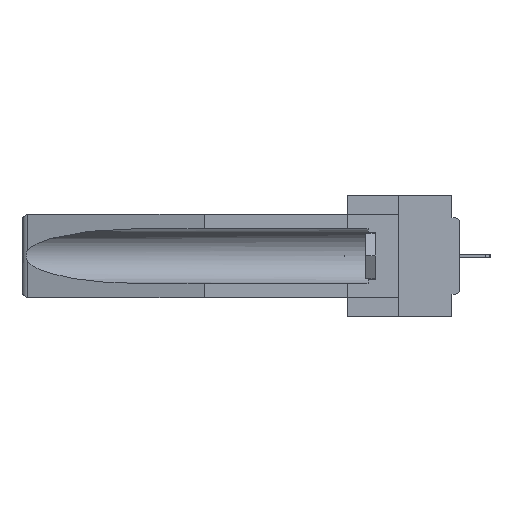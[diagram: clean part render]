
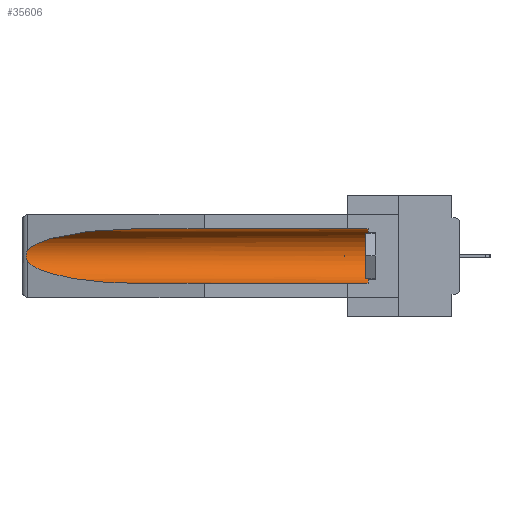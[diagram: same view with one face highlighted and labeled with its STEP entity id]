
A CAD part, left-side view. The second image highlights one B-rep face of the part: STEP entity #35606.
In plain terms, the highlighted cylindrical face has radius 2.857 mm (diameter 5.715 mm), a partial arc.
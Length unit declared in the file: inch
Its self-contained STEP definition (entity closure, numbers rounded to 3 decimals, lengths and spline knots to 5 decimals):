
#362 = ORIENTED_EDGE ( 'NONE', *, *, #18338, .F. ) ;
#703 = DIRECTION ( 'NONE',  ( 0., -1., 0. ) ) ;
#750 = CARTESIAN_POINT ( 'NONE',  ( 0.26537, 1.52718, -0.19328 ) ) ;
#1142 = DIRECTION ( 'NONE',  ( 0., 1., 0. ) ) ;
#1208 = DIRECTION ( 'NONE',  ( 0., 1., 0. ) ) ;
#2136 = EDGE_CURVE ( 'NONE', #2576, #16146, #40987, .T. ) ;
#2576 = VERTEX_POINT ( 'NONE', #750 ) ;
#3583 = CARTESIAN_POINT ( 'NONE',  ( 0.155, 0.126, -0.059 ) ) ;
#3843 = CARTESIAN_POINT ( 'NONE',  ( 0.25451, 1.48313, -0.24835 ) ) ;
#4377 = LINE ( 'NONE', #17209, #23886 ) ;
#4452 = CARTESIAN_POINT ( 'NONE',  ( 0.155, 1.07973, -0.284 ) ) ;
#5800 = CARTESIAN_POINT ( 'NONE',  ( 0.155, 1.07973, -0.059 ) ) ;
#6397 = ORIENTED_EDGE ( 'NONE', *, *, #2136, .T. ) ;
#6846 = EDGE_CURVE ( 'NONE', #24248, #17287, #15406, .T. ) ;
#8630 = CARTESIAN_POINT ( 'NONE',  ( 0.26654, 1.53092, -0.15636 ) ) ;
#8865 = CARTESIAN_POINT ( 'NONE',  ( 0.155, 0.126, -0.284 ) ) ;
#8889 = CARTESIAN_POINT ( 'NONE',  ( 0.26537, 1.52718, -0.14972 ) ) ;
#8976 = ORIENTED_EDGE ( 'NONE', *, *, #6846, .T. ) ;
#9620 = CARTESIAN_POINT ( 'NONE',  ( 0.155, -0.30754, -0.1715 ) ) ;
#9962 = DIRECTION ( 'NONE',  ( 0., 0., 1. ) ) ;
#10592 = CARTESIAN_POINT ( 'NONE',  ( 0.26537, 1.52718, -0.19328 ) ) ;
#12201 = CARTESIAN_POINT ( 'NONE',  ( 0.26537, 1.52718, -0.19328 ) ) ;
#12787 = ORIENTED_EDGE ( 'NONE', *, *, #16851, .T. ) ;
#13695 = VERTEX_POINT ( 'NONE', #3583 ) ;
#14252 = DIRECTION ( 'NONE',  ( 0., 1., 0. ) ) ;
#15339 = CARTESIAN_POINT ( 'NONE',  ( 0.26655, 1.53094, -0.18657 ) ) ;
#15406 =( BOUNDED_CURVE ( )  B_SPLINE_CURVE ( 3, ( #18164, #21319, #31427, #21098 ),
 .UNSPECIFIED., .F., .F. ) 
 B_SPLINE_CURVE_WITH_KNOTS ( ( 4, 4 ),
 ( 4.71239, 6.08839 ),
 .UNSPECIFIED. ) 
 CURVE ( )  GEOMETRIC_REPRESENTATION_ITEM ( )  RATIONAL_B_SPLINE_CURVE ( ( 1., 0.848, 0.848, 1. ) ) 
 REPRESENTATION_ITEM ( '' )  );
#16146 = VERTEX_POINT ( 'NONE', #21512 ) ;
#16598 = EDGE_CURVE ( 'NONE', #17287, #2576, #16915, .T. ) ;
#16851 = EDGE_CURVE ( 'NONE', #13695, #24248, #4377, .T. ) ;
#16915 = B_SPLINE_CURVE_WITH_KNOTS ( 'NONE', 3,
 ( #27775, #24613, #8630, #40818, #24827, #37648, #21654, #15339, #41042, #12201 ),
 .UNSPECIFIED., .F., .F.,
 ( 4, 2, 2, 2, 4 ),
 ( 0., 0.00029, 0.00058, 0.00087, 0.00117 ),
 .UNSPECIFIED. ) ;
#17209 = CARTESIAN_POINT ( 'NONE',  ( 0.155, -0.30754, -0.059 ) ) ;
#17287 = VERTEX_POINT ( 'NONE', #8889 ) ;
#17542 = EDGE_CURVE ( 'NONE', #31581, #13695, #35376, .T. ) ;
#18164 = CARTESIAN_POINT ( 'NONE',  ( 0.155, 1.07973, -0.059 ) ) ;
#18338 = EDGE_CURVE ( 'NONE', #31581, #16146, #23890, .T. ) ;
#20231 = CARTESIAN_POINT ( 'NONE',  ( 0.21114, 1.30732, -0.284 ) ) ;
#21098 = CARTESIAN_POINT ( 'NONE',  ( 0.26537, 1.52718, -0.14972 ) ) ;
#21319 = CARTESIAN_POINT ( 'NONE',  ( 0.21114, 1.30732, -0.059 ) ) ;
#21512 = CARTESIAN_POINT ( 'NONE',  ( 0.155, 1.07973, -0.284 ) ) ;
#21654 = CARTESIAN_POINT ( 'NONE',  ( 0.2673, 1.53269, -0.17917 ) ) ;
#22043 = ORIENTED_EDGE ( 'NONE', *, *, #17542, .T. ) ;
#22866 = FACE_OUTER_BOUND ( 'NONE', #30935, .T. ) ;
#23470 = AXIS2_PLACEMENT_3D ( 'NONE', #9620, #1142, #32111 ) ;
#23886 = VECTOR ( 'NONE', #14252, 39.37008 ) ;
#23890 = LINE ( 'NONE', #36718, #37302 ) ;
#24248 = VERTEX_POINT ( 'NONE', #5800 ) ;
#24613 = CARTESIAN_POINT ( 'NONE',  ( 0.26597, 1.52961, -0.15275 ) ) ;
#24827 = CARTESIAN_POINT ( 'NONE',  ( 0.2675, 1.53308, -0.16763 ) ) ;
#27775 = CARTESIAN_POINT ( 'NONE',  ( 0.26537, 1.52718, -0.14972 ) ) ;
#29283 = CARTESIAN_POINT ( 'NONE',  ( 0.155, 0.126, -0.1715 ) ) ;
#30179 = ORIENTED_EDGE ( 'NONE', *, *, #16598, .T. ) ;
#30935 = EDGE_LOOP ( 'NONE', ( #8976, #30179, #6397, #362, #22043, #12787 ) ) ;
#31427 = CARTESIAN_POINT ( 'NONE',  ( 0.25451, 1.48313, -0.09465 ) ) ;
#31581 = VERTEX_POINT ( 'NONE', #8865 ) ;
#32111 = DIRECTION ( 'NONE',  ( 0., 0., 1. ) ) ;
#32517 = CYLINDRICAL_SURFACE ( 'NONE', #23470, 0.1125 ) ;
#35376 = CIRCLE ( 'NONE', #41418, 0.1125 ) ;
#35606 = ADVANCED_FACE ( 'NONE', ( #22866 ), #32517, .F. ) ;
#36718 = CARTESIAN_POINT ( 'NONE',  ( 0.155, -0.30754, -0.284 ) ) ;
#37302 = VECTOR ( 'NONE', #1208, 39.37008 ) ;
#37648 = CARTESIAN_POINT ( 'NONE',  ( 0.2675, 1.53308, -0.17534 ) ) ;
#40818 = CARTESIAN_POINT ( 'NONE',  ( 0.2673, 1.5327, -0.16383 ) ) ;
#40987 =( BOUNDED_CURVE ( )  B_SPLINE_CURVE ( 3, ( #10592, #3843, #20231, #4452 ),
 .UNSPECIFIED., .F., .F. ) 
 B_SPLINE_CURVE_WITH_KNOTS ( ( 4, 4 ),
 ( 0.1948, 1.5708 ),
 .UNSPECIFIED. ) 
 CURVE ( )  GEOMETRIC_REPRESENTATION_ITEM ( )  RATIONAL_B_SPLINE_CURVE ( ( 1., 0.848, 0.848, 1. ) ) 
 REPRESENTATION_ITEM ( '' )  );
#41042 = CARTESIAN_POINT ( 'NONE',  ( 0.26597, 1.5296, -0.19026 ) ) ;
#41418 = AXIS2_PLACEMENT_3D ( 'NONE', #29283, #703, #9962 ) ;
